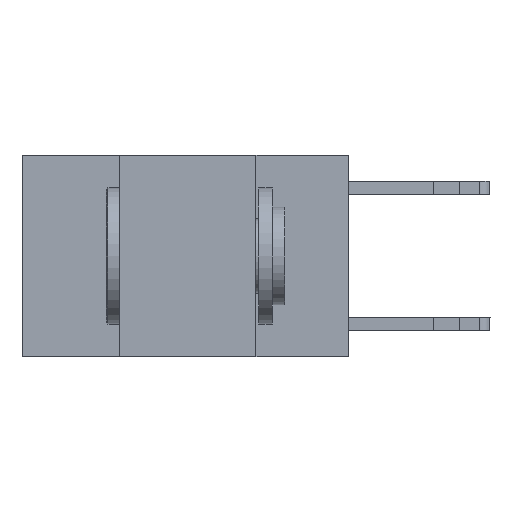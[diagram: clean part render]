
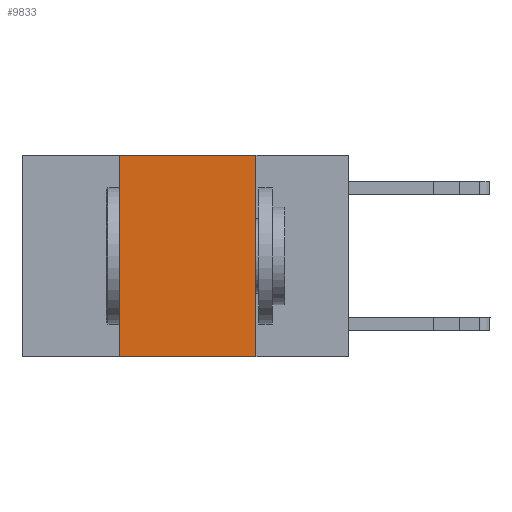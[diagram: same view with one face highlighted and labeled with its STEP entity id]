
A CAD part, left-side view. The second image highlights one B-rep face of the part: STEP entity #9833.
In plain terms, the highlighted planar face has unit normal (-1, 0, 0).
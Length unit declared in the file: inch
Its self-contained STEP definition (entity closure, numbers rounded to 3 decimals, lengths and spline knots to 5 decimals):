
#90 = DIRECTION ( 'NONE',  ( 0., 0., 1. ) ) ;
#311 = LINE ( 'NONE', #11385, #1222 ) ;
#606 = EDGE_CURVE ( 'NONE', #4802, #4003, #311, .T. ) ;
#627 = CARTESIAN_POINT ( 'NONE',  ( 0., 0.17, -0.37 ) ) ;
#1222 = VECTOR ( 'NONE', #4489, 39.37008 ) ;
#1317 = VERTEX_POINT ( 'NONE', #5643 ) ;
#1336 = VECTOR ( 'NONE', #8793, 39.37008 ) ;
#1375 = PLANE ( 'NONE',  #12078 ) ;
#1839 = DIRECTION ( 'NONE',  ( 1., 0., 0. ) ) ;
#2477 = DIRECTION ( 'NONE',  ( 0., 0., -1. ) ) ;
#2614 = CARTESIAN_POINT ( 'NONE',  ( 0., 0.17, 0. ) ) ;
#2839 = ORIENTED_EDGE ( 'NONE', *, *, #11134, .F. ) ;
#3437 = VECTOR ( 'NONE', #90, 39.37008 ) ;
#3959 = ORIENTED_EDGE ( 'NONE', *, *, #8556, .F. ) ;
#4003 = VERTEX_POINT ( 'NONE', #627 ) ;
#4489 = DIRECTION ( 'NONE',  ( 0., -1., 0. ) ) ;
#4637 = CARTESIAN_POINT ( 'NONE',  ( 0., 0.6, 0. ) ) ;
#4658 = LINE ( 'NONE', #2614, #9574 ) ;
#4782 = LINE ( 'NONE', #4637, #1336 ) ;
#4802 = VERTEX_POINT ( 'NONE', #6590 ) ;
#4957 = CARTESIAN_POINT ( 'NONE',  ( 0., 0.6, 0. ) ) ;
#5643 = CARTESIAN_POINT ( 'NONE',  ( 0., 0.17, 0. ) ) ;
#5975 = EDGE_CURVE ( 'NONE', #10581, #1317, #4782, .T. ) ;
#6590 = CARTESIAN_POINT ( 'NONE',  ( 0., 0.42, -0.37 ) ) ;
#8531 = CARTESIAN_POINT ( 'NONE',  ( 0., 0.42, 0. ) ) ;
#8556 = EDGE_CURVE ( 'NONE', #4802, #10581, #9863, .T. ) ;
#8793 = DIRECTION ( 'NONE',  ( 0., -1., 0. ) ) ;
#8866 = ORIENTED_EDGE ( 'NONE', *, *, #5975, .F. ) ;
#9348 = EDGE_LOOP ( 'NONE', ( #2839, #8866, #3959, #9510 ) ) ;
#9510 = ORIENTED_EDGE ( 'NONE', *, *, #606, .T. ) ;
#9574 = VECTOR ( 'NONE', #2477, 39.37008 ) ;
#9833 = ADVANCED_FACE ( 'NONE', ( #12370 ), #1375, .F. ) ;
#9863 = LINE ( 'NONE', #12115, #3437 ) ;
#10581 = VERTEX_POINT ( 'NONE', #8531 ) ;
#11134 = EDGE_CURVE ( 'NONE', #1317, #4003, #4658, .T. ) ;
#11385 = CARTESIAN_POINT ( 'NONE',  ( 0., 0.6, -0.37 ) ) ;
#12049 = DIRECTION ( 'NONE',  ( 0., 0., -1. ) ) ;
#12078 = AXIS2_PLACEMENT_3D ( 'NONE', #4957, #1839, #12049 ) ;
#12115 = CARTESIAN_POINT ( 'NONE',  ( 0., 0.42, 0. ) ) ;
#12370 = FACE_OUTER_BOUND ( 'NONE', #9348, .T. ) ;
